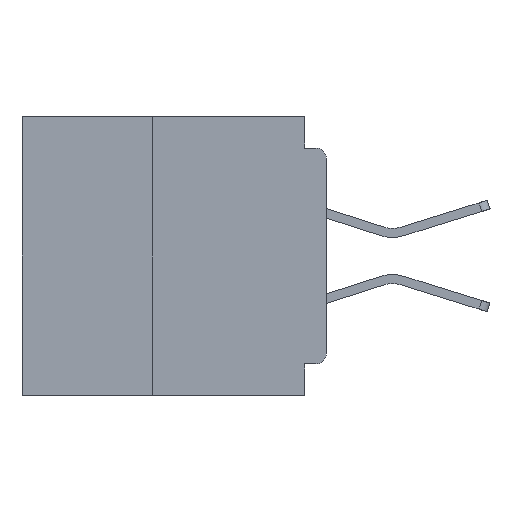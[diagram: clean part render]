
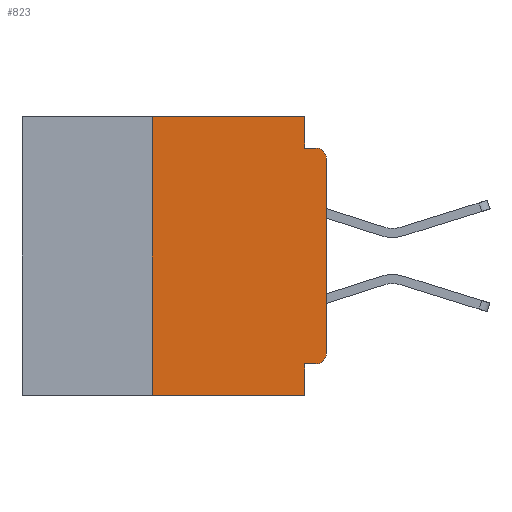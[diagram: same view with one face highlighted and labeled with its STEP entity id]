
A CAD part, left-side view. The second image highlights one B-rep face of the part: STEP entity #823.
In plain terms, the highlighted planar face has unit normal (-1, 0, 0).
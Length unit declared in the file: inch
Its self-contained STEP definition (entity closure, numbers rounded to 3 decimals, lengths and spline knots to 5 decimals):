
#759 = EDGE_CURVE ( 'NONE', #45184, #37290, #18157, .T. ) ;
#823 = ADVANCED_FACE ( 'NONE', ( #51200 ), #48165, .F. ) ;
#1358 = CARTESIAN_POINT ( 'NONE',  ( 0., 0.031, -0.045 ) ) ;
#2157 = DIRECTION ( 'NONE',  ( 0., 1., 0. ) ) ;
#2277 = VECTOR ( 'NONE', #50240, 39.37008 ) ;
#3016 = VECTOR ( 'NONE', #28514, 39.37008 ) ;
#3086 = CARTESIAN_POINT ( 'NONE',  ( 0., 0.015, -0.355 ) ) ;
#4940 = VERTEX_POINT ( 'NONE', #41407 ) ;
#5659 = DIRECTION ( 'NONE',  ( 1., 0., 0. ) ) ;
#5700 = ORIENTED_EDGE ( 'NONE', *, *, #759, .F. ) ;
#5791 = VECTOR ( 'NONE', #38365, 39.37008 ) ;
#6584 = DIRECTION ( 'NONE',  ( 0., 0., -1. ) ) ;
#6692 = ORIENTED_EDGE ( 'NONE', *, *, #54174, .T. ) ;
#7292 = EDGE_CURVE ( 'NONE', #59320, #23797, #48618, .T. ) ;
#14599 = AXIS2_PLACEMENT_3D ( 'NONE', #22260, #55698, #27070 ) ;
#15644 = ORIENTED_EDGE ( 'NONE', *, *, #51966, .T. ) ;
#15711 = VERTEX_POINT ( 'NONE', #17160 ) ;
#16973 = CARTESIAN_POINT ( 'NONE',  ( 0., 0.437, -0.4 ) ) ;
#17160 = CARTESIAN_POINT ( 'NONE',  ( 0., 0.25, -0.4 ) ) ;
#18157 = LINE ( 'NONE', #37679, #2277 ) ;
#18397 = LINE ( 'NONE', #32775, #40932 ) ;
#18762 = CARTESIAN_POINT ( 'NONE',  ( 0., 0.031, 0. ) ) ;
#20151 = DIRECTION ( 'NONE',  ( 0., 0., -1. ) ) ;
#20874 = CARTESIAN_POINT ( 'NONE',  ( 0., 0.031, 0. ) ) ;
#22260 = CARTESIAN_POINT ( 'NONE',  ( 0., 0.015, -0.34 ) ) ;
#22272 = LINE ( 'NONE', #45255, #46241 ) ;
#23124 = VECTOR ( 'NONE', #44582, 39.37008 ) ;
#23693 = CARTESIAN_POINT ( 'NONE',  ( 0., 0.25, -0.4 ) ) ;
#23797 = VERTEX_POINT ( 'NONE', #54308 ) ;
#25052 = CARTESIAN_POINT ( 'NONE',  ( 0., 0.437, 0. ) ) ;
#25628 = LINE ( 'NONE', #23693, #3016 ) ;
#25648 = VERTEX_POINT ( 'NONE', #45683 ) ;
#27046 = DIRECTION ( 'NONE',  ( -1., 0., 0. ) ) ;
#27070 = DIRECTION ( 'NONE',  ( 0., 0., -1. ) ) ;
#27621 = ORIENTED_EDGE ( 'NONE', *, *, #52346, .T. ) ;
#28514 = DIRECTION ( 'NONE',  ( 0., 0., 1. ) ) ;
#29163 = AXIS2_PLACEMENT_3D ( 'NONE', #25052, #5659, #20151 ) ;
#31591 = LINE ( 'NONE', #16973, #56998 ) ;
#32391 = ORIENTED_EDGE ( 'NONE', *, *, #36442, .T. ) ;
#32620 = CIRCLE ( 'NONE', #48418, 0.015 ) ;
#32775 = CARTESIAN_POINT ( 'NONE',  ( 0., 0., 0. ) ) ;
#34987 = VECTOR ( 'NONE', #6584, 39.37008 ) ;
#35596 = ORIENTED_EDGE ( 'NONE', *, *, #46042, .F. ) ;
#36442 = EDGE_CURVE ( 'NONE', #25648, #23797, #32620, .T. ) ;
#36519 = EDGE_LOOP ( 'NONE', ( #15644, #32391, #37032, #41229, #5700, #53605, #6692, #35596, #46537, #27621 ) ) ;
#37032 = ORIENTED_EDGE ( 'NONE', *, *, #7292, .F. ) ;
#37290 = VERTEX_POINT ( 'NONE', #18762 ) ;
#37679 = CARTESIAN_POINT ( 'NONE',  ( 0., 0.437, 0. ) ) ;
#38001 = LINE ( 'NONE', #20874, #34987 ) ;
#38365 = DIRECTION ( 'NONE',  ( 0., 0., -1. ) ) ;
#39375 = VERTEX_POINT ( 'NONE', #51927 ) ;
#40932 = VECTOR ( 'NONE', #61568, 39.37008 ) ;
#41214 = EDGE_CURVE ( 'NONE', #15711, #45184, #25628, .T. ) ;
#41229 = ORIENTED_EDGE ( 'NONE', *, *, #45043, .F. ) ;
#41407 = CARTESIAN_POINT ( 'NONE',  ( 0., 0.031, -0.4 ) ) ;
#44582 = DIRECTION ( 'NONE',  ( 0., -1., 0. ) ) ;
#44813 = CARTESIAN_POINT ( 'NONE',  ( 0., 0., -0.34 ) ) ;
#45043 = EDGE_CURVE ( 'NONE', #37290, #59320, #38001, .T. ) ;
#45184 = VERTEX_POINT ( 'NONE', #45763 ) ;
#45255 = CARTESIAN_POINT ( 'NONE',  ( 0., 0., -0.355 ) ) ;
#45683 = CARTESIAN_POINT ( 'NONE',  ( 0., 0., -0.06 ) ) ;
#45763 = CARTESIAN_POINT ( 'NONE',  ( 0., 0.25, 0. ) ) ;
#46042 = EDGE_CURVE ( 'NONE', #39375, #4940, #58242, .T. ) ;
#46241 = VECTOR ( 'NONE', #2157, 39.37008 ) ;
#46300 = VERTEX_POINT ( 'NONE', #44813 ) ;
#46537 = ORIENTED_EDGE ( 'NONE', *, *, #56588, .F. ) ;
#48165 = PLANE ( 'NONE',  #29163 ) ;
#48418 = AXIS2_PLACEMENT_3D ( 'NONE', #55675, #27046, #60487 ) ;
#48618 = LINE ( 'NONE', #58751, #23124 ) ;
#50240 = DIRECTION ( 'NONE',  ( 0., -1., 0. ) ) ;
#50487 = DIRECTION ( 'NONE',  ( 0., -1., 0. ) ) ;
#51200 = FACE_OUTER_BOUND ( 'NONE', #36519, .T. ) ;
#51927 = CARTESIAN_POINT ( 'NONE',  ( 0., 0.031, -0.355 ) ) ;
#51966 = EDGE_CURVE ( 'NONE', #46300, #25648, #18397, .T. ) ;
#52346 = EDGE_CURVE ( 'NONE', #56036, #46300, #56508, .T. ) ;
#52754 = CARTESIAN_POINT ( 'NONE',  ( 0., 0.031, -0.4 ) ) ;
#53605 = ORIENTED_EDGE ( 'NONE', *, *, #41214, .F. ) ;
#54174 = EDGE_CURVE ( 'NONE', #15711, #4940, #31591, .T. ) ;
#54308 = CARTESIAN_POINT ( 'NONE',  ( 0., 0.015, -0.045 ) ) ;
#55675 = CARTESIAN_POINT ( 'NONE',  ( 0., 0.015, -0.06 ) ) ;
#55698 = DIRECTION ( 'NONE',  ( -1., 0., 0. ) ) ;
#56036 = VERTEX_POINT ( 'NONE', #3086 ) ;
#56508 = CIRCLE ( 'NONE', #14599, 0.015 ) ;
#56588 = EDGE_CURVE ( 'NONE', #56036, #39375, #22272, .T. ) ;
#56998 = VECTOR ( 'NONE', #50487, 39.37008 ) ;
#58242 = LINE ( 'NONE', #52754, #5791 ) ;
#58751 = CARTESIAN_POINT ( 'NONE',  ( 0., 0., -0.045 ) ) ;
#59320 = VERTEX_POINT ( 'NONE', #1358 ) ;
#60487 = DIRECTION ( 'NONE',  ( 0., 0., -1. ) ) ;
#61568 = DIRECTION ( 'NONE',  ( 0., 0., 1. ) ) ;
